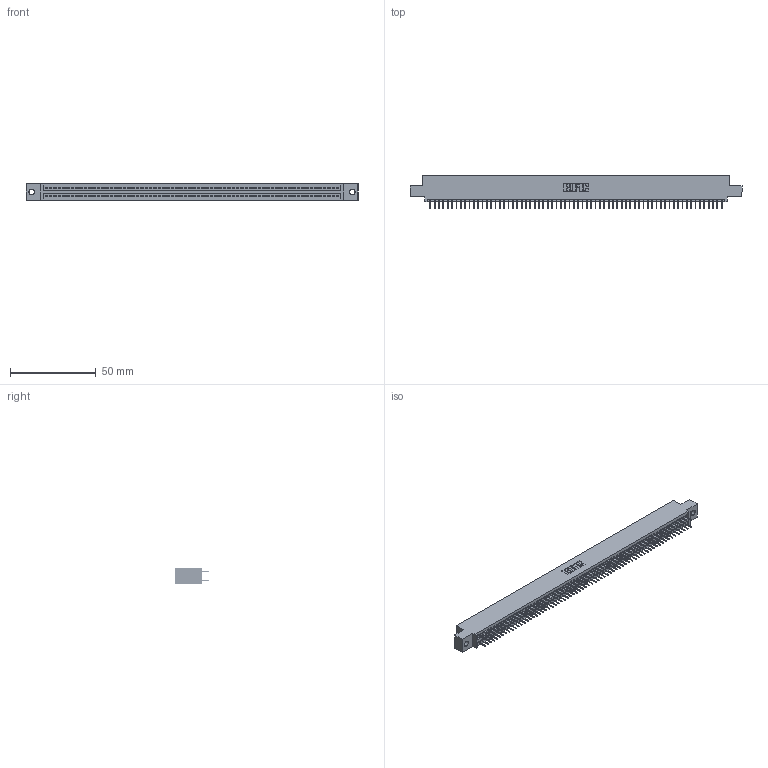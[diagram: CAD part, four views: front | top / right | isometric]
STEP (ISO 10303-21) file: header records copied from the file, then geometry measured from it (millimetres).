
FILE_DESCRIPTION (( 'STEP AP203' ), '1' );
FILE_NAME ('395-136-524-502.STEP', '2019-10-29T15:43:30', ( '' ), ( '' ), 'SwSTEP 2.0', 'SolidWorks 2016', '' );
FILE_SCHEMA (( 'CONFIG_CONTROL_DESIGN' ));
Length unit declared in the file: inch
Products named in the file (3): 395-136-524-502; 345 Part_0.110 Offset - 0.128 Dia; 345-292-001_345-293-124
Assembly tree (137 placements, depth 2):
  395-136-524-502
    345 Part_0.110 Offset - 0.128 Dia
    345-292-001_345-293-124  x136
Bounding box: 193.93 x 19.35 x 9.4 mm (x, y, z)
Volume: 18763.9 mm3; surface area: 27516.6 mm2
Topology: 137 solids, 137 shells, 7474 faces, 21161 edges, 13562 vertices
Faces by surface type: plane 5388, cylinder 2086
Entity records: 50063 total; most frequent: CARTESIAN_POINT 8368, ORIENTED_EDGE 8302, DIRECTION 7347, EDGE_CURVE 4151, VECTOR 3751, LINE 3751, VERTEX_POINT 2762, AXIS2_PLACEMENT_3D 1798
